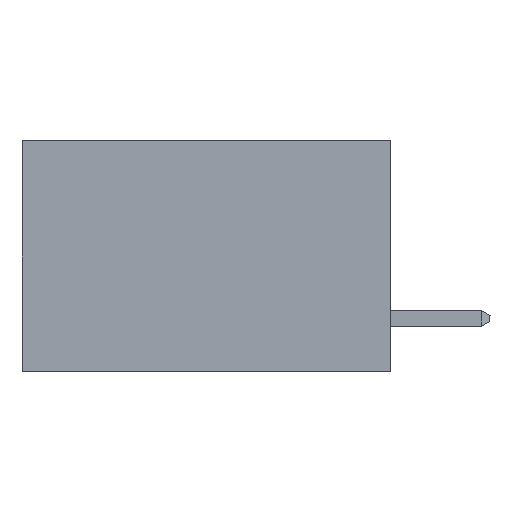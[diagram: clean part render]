
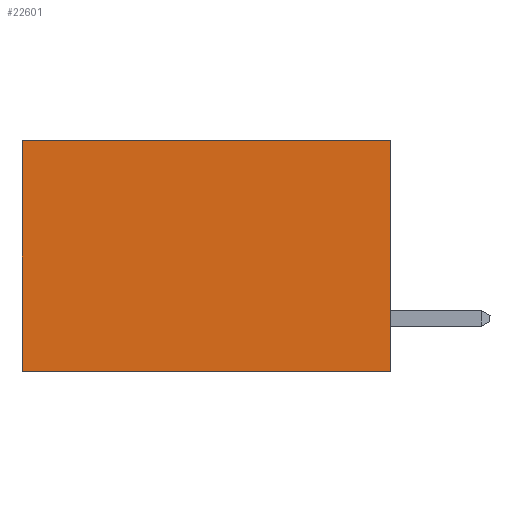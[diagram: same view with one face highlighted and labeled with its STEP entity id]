
A CAD part, left-side view. The second image highlights one B-rep face of the part: STEP entity #22601.
In plain terms, the highlighted planar face has unit normal (-1, 0, 0).
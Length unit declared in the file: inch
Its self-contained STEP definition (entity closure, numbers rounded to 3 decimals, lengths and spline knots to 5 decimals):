
#813 = DIRECTION ( 'NONE',  ( 0., 0., -1. ) ) ;
#2332 = DIRECTION ( 'NONE',  ( 0., 1., 0. ) ) ;
#2968 = CARTESIAN_POINT ( 'NONE',  ( 0.277, 0.59, 0. ) ) ;
#3879 = EDGE_CURVE ( 'NONE', #9654, #11476, #22117, .T. ) ;
#4307 = ORIENTED_EDGE ( 'NONE', *, *, #4961, .T. ) ;
#4390 = ORIENTED_EDGE ( 'NONE', *, *, #3879, .F. ) ;
#4673 = ORIENTED_EDGE ( 'NONE', *, *, #25834, .F. ) ;
#4701 = ORIENTED_EDGE ( 'NONE', *, *, #21517, .T. ) ;
#4779 = AXIS2_PLACEMENT_3D ( 'NONE', #17445, #5171, #22324 ) ;
#4961 = EDGE_CURVE ( 'NONE', #23891, #11476, #28119, .T. ) ;
#5171 = DIRECTION ( 'NONE',  ( 1., 0., 0. ) ) ;
#5774 = CARTESIAN_POINT ( 'NONE',  ( 0.277, 0., -0.37 ) ) ;
#6980 = VECTOR ( 'NONE', #813, 39.37008 ) ;
#8692 = EDGE_LOOP ( 'NONE', ( #4307, #4390, #4673, #4701 ) ) ;
#9056 = VECTOR ( 'NONE', #2332, 39.37008 ) ;
#9654 = VERTEX_POINT ( 'NONE', #5774 ) ;
#11272 = VECTOR ( 'NONE', #30754, 39.37008 ) ;
#11476 = VERTEX_POINT ( 'NONE', #27124 ) ;
#13539 = LINE ( 'NONE', #22881, #6980 ) ;
#13804 = CARTESIAN_POINT ( 'NONE',  ( 0.277, 0., 0. ) ) ;
#17445 = CARTESIAN_POINT ( 'NONE',  ( 0.277, 0., -0.37 ) ) ;
#17836 = FACE_OUTER_BOUND ( 'NONE', #8692, .T. ) ;
#18695 = VERTEX_POINT ( 'NONE', #23641 ) ;
#18789 = CARTESIAN_POINT ( 'NONE',  ( 0.277, 0.59, -0.37 ) ) ;
#19875 = PLANE ( 'NONE',  #4779 ) ;
#20891 = VECTOR ( 'NONE', #21326, 39.37008 ) ;
#21326 = DIRECTION ( 'NONE',  ( 0., 0., -1. ) ) ;
#21517 = EDGE_CURVE ( 'NONE', #18695, #23891, #30675, .T. ) ;
#22117 = LINE ( 'NONE', #23384, #9056 ) ;
#22324 = DIRECTION ( 'NONE',  ( 0., 0., -1. ) ) ;
#22601 = ADVANCED_FACE ( 'NONE', ( #17836 ), #19875, .F. ) ;
#22881 = CARTESIAN_POINT ( 'NONE',  ( 0.277, 0., -0.37 ) ) ;
#23384 = CARTESIAN_POINT ( 'NONE',  ( 0.277, 0., -0.37 ) ) ;
#23641 = CARTESIAN_POINT ( 'NONE',  ( 0.277, 0., 0. ) ) ;
#23891 = VERTEX_POINT ( 'NONE', #2968 ) ;
#25834 = EDGE_CURVE ( 'NONE', #18695, #9654, #13539, .T. ) ;
#27124 = CARTESIAN_POINT ( 'NONE',  ( 0.277, 0.59, -0.37 ) ) ;
#28119 = LINE ( 'NONE', #18789, #20891 ) ;
#30675 = LINE ( 'NONE', #13804, #11272 ) ;
#30754 = DIRECTION ( 'NONE',  ( 0., 1., 0. ) ) ;
